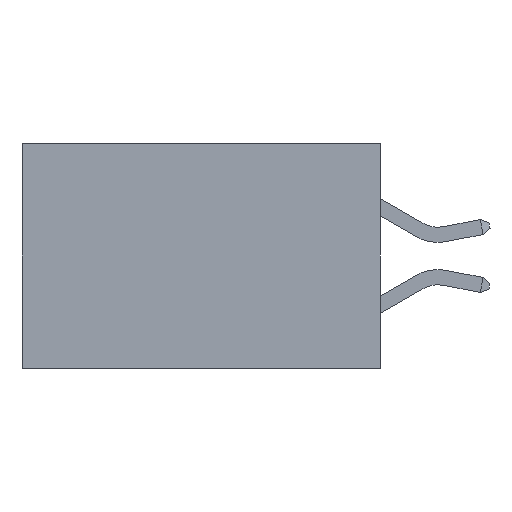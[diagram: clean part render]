
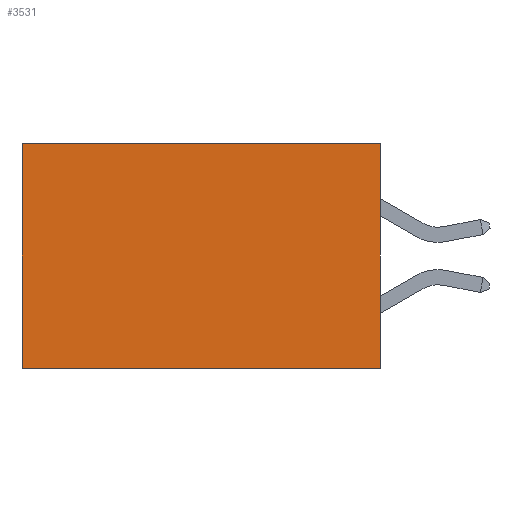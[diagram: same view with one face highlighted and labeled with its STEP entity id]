
A CAD part, left-side view. The second image highlights one B-rep face of the part: STEP entity #3531.
In plain terms, the highlighted planar face has unit normal (-1, 0, 0).
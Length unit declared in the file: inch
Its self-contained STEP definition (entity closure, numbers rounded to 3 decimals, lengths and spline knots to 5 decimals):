
#913 = EDGE_LOOP ( 'NONE', ( #6133, #6972, #7685, #11555 ) ) ;
#2473 = EDGE_CURVE ( 'NONE', #15098, #8116, #17868, .T. ) ;
#2847 = LINE ( 'NONE', #6433, #13045 ) ;
#3531 = ADVANCED_FACE ( 'NONE', ( #6624 ), #16748, .F. ) ;
#4937 = CARTESIAN_POINT ( 'NONE',  ( 0.277, 0.59, 0. ) ) ;
#5628 = EDGE_CURVE ( 'NONE', #15098, #9243, #2847, .T. ) ;
#6097 = AXIS2_PLACEMENT_3D ( 'NONE', #16731, #6244, #6484 ) ;
#6133 = ORIENTED_EDGE ( 'NONE', *, *, #10163, .T. ) ;
#6244 = DIRECTION ( 'NONE',  ( 1., 0., 0. ) ) ;
#6433 = CARTESIAN_POINT ( 'NONE',  ( 0.277, 0., 0. ) ) ;
#6484 = DIRECTION ( 'NONE',  ( 0., 0., -1. ) ) ;
#6624 = FACE_OUTER_BOUND ( 'NONE', #913, .T. ) ;
#6719 = VECTOR ( 'NONE', #8848, 39.37008 ) ;
#6731 = LINE ( 'NONE', #15779, #13643 ) ;
#6942 = DIRECTION ( 'NONE',  ( 0., 1., 0. ) ) ;
#6972 = ORIENTED_EDGE ( 'NONE', *, *, #7148, .F. ) ;
#7148 = EDGE_CURVE ( 'NONE', #8116, #9846, #6731, .T. ) ;
#7685 = ORIENTED_EDGE ( 'NONE', *, *, #2473, .F. ) ;
#8116 = VERTEX_POINT ( 'NONE', #12020 ) ;
#8611 = LINE ( 'NONE', #13142, #11813 ) ;
#8691 = DIRECTION ( 'NONE',  ( 0., 1., 0. ) ) ;
#8848 = DIRECTION ( 'NONE',  ( 0., 0., -1. ) ) ;
#8864 = CARTESIAN_POINT ( 'NONE',  ( 0.277, 0., -0.37 ) ) ;
#8997 = CARTESIAN_POINT ( 'NONE',  ( 0.277, 0., 0. ) ) ;
#9243 = VERTEX_POINT ( 'NONE', #4937 ) ;
#9846 = VERTEX_POINT ( 'NONE', #17522 ) ;
#10163 = EDGE_CURVE ( 'NONE', #9243, #9846, #8611, .T. ) ;
#11555 = ORIENTED_EDGE ( 'NONE', *, *, #5628, .T. ) ;
#11813 = VECTOR ( 'NONE', #13161, 39.37008 ) ;
#12020 = CARTESIAN_POINT ( 'NONE',  ( 0.277, 0., -0.37 ) ) ;
#13045 = VECTOR ( 'NONE', #6942, 39.37008 ) ;
#13142 = CARTESIAN_POINT ( 'NONE',  ( 0.277, 0.59, -0.37 ) ) ;
#13161 = DIRECTION ( 'NONE',  ( 0., 0., -1. ) ) ;
#13643 = VECTOR ( 'NONE', #8691, 39.37008 ) ;
#15098 = VERTEX_POINT ( 'NONE', #8997 ) ;
#15779 = CARTESIAN_POINT ( 'NONE',  ( 0.277, 0., -0.37 ) ) ;
#16731 = CARTESIAN_POINT ( 'NONE',  ( 0.277, 0., -0.37 ) ) ;
#16748 = PLANE ( 'NONE',  #6097 ) ;
#17522 = CARTESIAN_POINT ( 'NONE',  ( 0.277, 0.59, -0.37 ) ) ;
#17868 = LINE ( 'NONE', #8864, #6719 ) ;
